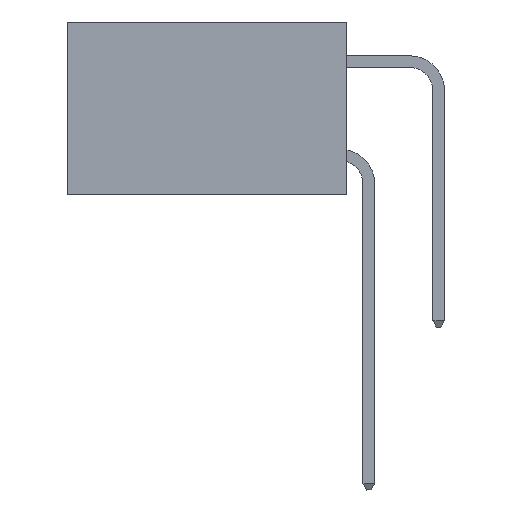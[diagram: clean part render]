
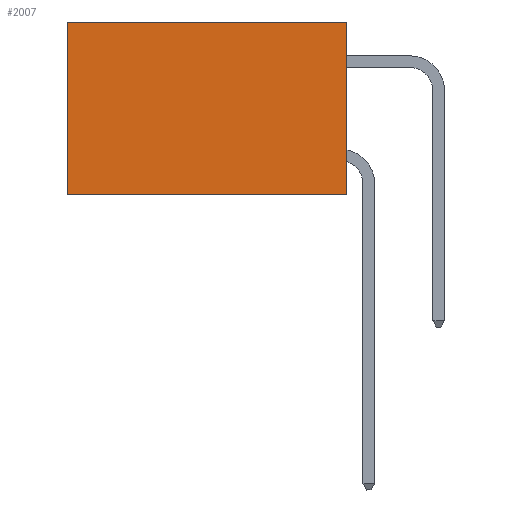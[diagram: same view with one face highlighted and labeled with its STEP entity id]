
A CAD part, left-side view. The second image highlights one B-rep face of the part: STEP entity #2007.
In plain terms, the highlighted planar face has unit normal (-1, 0, 0).
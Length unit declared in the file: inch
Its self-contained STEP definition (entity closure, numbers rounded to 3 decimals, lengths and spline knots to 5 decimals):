
#333 = CARTESIAN_POINT ( 'NONE',  ( 0.2875, 0., 0. ) ) ;
#1171 = ORIENTED_EDGE ( 'NONE', *, *, #21314, .F. ) ;
#2007 = ADVANCED_FACE ( 'NONE', ( #6568 ), #26887, .F. ) ;
#2201 = CARTESIAN_POINT ( 'NONE',  ( 0.2875, 0.6, -0.37 ) ) ;
#2391 = EDGE_LOOP ( 'NONE', ( #17677, #1171, #14996, #38531 ) ) ;
#2701 = VECTOR ( 'NONE', #26814, 39.37008 ) ;
#3710 = CARTESIAN_POINT ( 'NONE',  ( 0.2875, 0.6, 0. ) ) ;
#4108 = DIRECTION ( 'NONE',  ( 1., 0., 0. ) ) ;
#6568 = FACE_OUTER_BOUND ( 'NONE', #2391, .T. ) ;
#7029 = EDGE_CURVE ( 'NONE', #39082, #34042, #38690, .T. ) ;
#10041 = CARTESIAN_POINT ( 'NONE',  ( 0.2875, 0., -0.37 ) ) ;
#10406 = CARTESIAN_POINT ( 'NONE',  ( 0.2875, 0., 0. ) ) ;
#10665 = VERTEX_POINT ( 'NONE', #3710 ) ;
#11644 = CARTESIAN_POINT ( 'NONE',  ( 0.2875, 0., 0. ) ) ;
#12774 = LINE ( 'NONE', #10041, #37562 ) ;
#13964 = VECTOR ( 'NONE', #34367, 39.37008 ) ;
#14996 = ORIENTED_EDGE ( 'NONE', *, *, #7029, .F. ) ;
#16275 = DIRECTION ( 'NONE',  ( 0., 0., -1. ) ) ;
#17093 = EDGE_CURVE ( 'NONE', #39082, #10665, #36435, .T. ) ;
#17677 = ORIENTED_EDGE ( 'NONE', *, *, #19602, .T. ) ;
#18635 = VECTOR ( 'NONE', #16275, 39.37008 ) ;
#19602 = EDGE_CURVE ( 'NONE', #10665, #24797, #34749, .T. ) ;
#21314 = EDGE_CURVE ( 'NONE', #34042, #24797, #12774, .T. ) ;
#24182 = AXIS2_PLACEMENT_3D ( 'NONE', #333, #4108, #32160 ) ;
#24797 = VERTEX_POINT ( 'NONE', #2201 ) ;
#26814 = DIRECTION ( 'NONE',  ( 0., 1., 0. ) ) ;
#26887 = PLANE ( 'NONE',  #24182 ) ;
#29673 = DIRECTION ( 'NONE',  ( 0., 1., 0. ) ) ;
#32090 = CARTESIAN_POINT ( 'NONE',  ( 0.2875, 0., 0. ) ) ;
#32160 = DIRECTION ( 'NONE',  ( 0., 0., -1. ) ) ;
#33946 = CARTESIAN_POINT ( 'NONE',  ( 0.2875, 0., -0.37 ) ) ;
#34042 = VERTEX_POINT ( 'NONE', #33946 ) ;
#34367 = DIRECTION ( 'NONE',  ( 0., 0., -1. ) ) ;
#34749 = LINE ( 'NONE', #35611, #18635 ) ;
#35611 = CARTESIAN_POINT ( 'NONE',  ( 0.2875, 0.6, 0. ) ) ;
#36435 = LINE ( 'NONE', #10406, #2701 ) ;
#37562 = VECTOR ( 'NONE', #29673, 39.37008 ) ;
#38531 = ORIENTED_EDGE ( 'NONE', *, *, #17093, .T. ) ;
#38690 = LINE ( 'NONE', #11644, #13964 ) ;
#39082 = VERTEX_POINT ( 'NONE', #32090 ) ;
